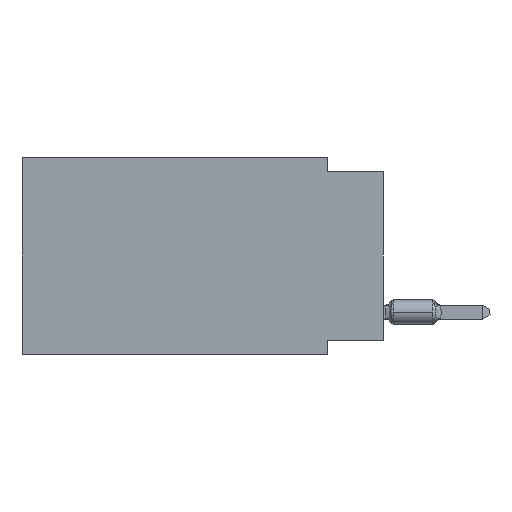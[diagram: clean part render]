
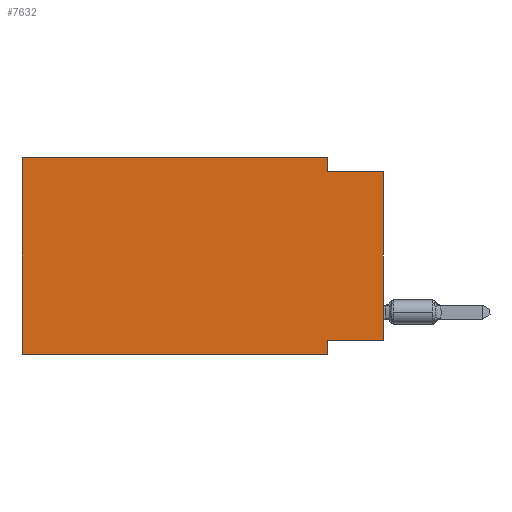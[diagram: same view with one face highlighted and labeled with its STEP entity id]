
A CAD part, left-side view. The second image highlights one B-rep face of the part: STEP entity #7632.
In plain terms, the highlighted planar face has unit normal (-1, 0, 0).
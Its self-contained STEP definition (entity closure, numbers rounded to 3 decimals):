
#23 = EDGE_CURVE ( 'NONE', #9929, #15581, #19994, .T. ) ;
#679 = ORIENTED_EDGE ( 'NONE', *, *, #10187, .F. ) ;
#808 = VECTOR ( 'NONE', #7598, 1000. ) ;
#1377 = ORIENTED_EDGE ( 'NONE', *, *, #15057, .F. ) ;
#1378 = LINE ( 'NONE', #15219, #3775 ) ;
#1688 = CARTESIAN_POINT ( 'NONE',  ( 0., 0., -8.255 ) ) ;
#1739 = VECTOR ( 'NONE', #7626, 1000. ) ;
#1839 = EDGE_CURVE ( 'NONE', #20794, #7504, #7367, .T. ) ;
#2128 = VECTOR ( 'NONE', #15510, 1000. ) ;
#2418 = LINE ( 'NONE', #11044, #1739 ) ;
#3391 = DIRECTION ( 'NONE',  ( 1., 0., 0. ) ) ;
#3775 = VECTOR ( 'NONE', #20628, 1000. ) ;
#4055 = CARTESIAN_POINT ( 'NONE',  ( 0., 2.54, 0. ) ) ;
#4470 = CARTESIAN_POINT ( 'NONE',  ( 0., 2.54, -8.89 ) ) ;
#5055 = DIRECTION ( 'NONE',  ( 0., 0., -1. ) ) ;
#5067 = CARTESIAN_POINT ( 'NONE',  ( 0., 16.383, 0. ) ) ;
#5190 = PLANE ( 'NONE',  #21615 ) ;
#5310 = EDGE_CURVE ( 'NONE', #8662, #15581, #6787, .T. ) ;
#5370 = VERTEX_POINT ( 'NONE', #14698 ) ;
#5507 = VECTOR ( 'NONE', #5919, 1000. ) ;
#5919 = DIRECTION ( 'NONE',  ( 0., 1., 0. ) ) ;
#6044 = EDGE_CURVE ( 'NONE', #9859, #20794, #20793, .T. ) ;
#6668 = CARTESIAN_POINT ( 'NONE',  ( 0., 2.54, -8.89 ) ) ;
#6787 = LINE ( 'NONE', #10658, #808 ) ;
#7367 = LINE ( 'NONE', #9318, #22335 ) ;
#7504 = VERTEX_POINT ( 'NONE', #9598 ) ;
#7598 = DIRECTION ( 'NONE',  ( 0., -1., 0. ) ) ;
#7626 = DIRECTION ( 'NONE',  ( 0., 0., 1. ) ) ;
#7632 = ADVANCED_FACE ( 'NONE', ( #22309 ), #5190, .F. ) ;
#8662 = VERTEX_POINT ( 'NONE', #16395 ) ;
#8968 = VECTOR ( 'NONE', #5055, 1000. ) ;
#9025 = EDGE_CURVE ( 'NONE', #22347, #7504, #2418, .T. ) ;
#9310 = VECTOR ( 'NONE', #19646, 1000. ) ;
#9318 = CARTESIAN_POINT ( 'NONE',  ( 0., 0., -0.635 ) ) ;
#9598 = CARTESIAN_POINT ( 'NONE',  ( 0., 0., -0.635 ) ) ;
#9849 = ORIENTED_EDGE ( 'NONE', *, *, #1839, .F. ) ;
#9859 = VERTEX_POINT ( 'NONE', #4055 ) ;
#9929 = VERTEX_POINT ( 'NONE', #18569 ) ;
#10187 = EDGE_CURVE ( 'NONE', #8662, #5370, #12223, .T. ) ;
#10658 = CARTESIAN_POINT ( 'NONE',  ( 0., 16.383, -8.89 ) ) ;
#11044 = CARTESIAN_POINT ( 'NONE',  ( 0., 0., 0. ) ) ;
#12223 = LINE ( 'NONE', #5067, #2128 ) ;
#12614 = DIRECTION ( 'NONE',  ( 0., -1., 0. ) ) ;
#13385 = CARTESIAN_POINT ( 'NONE',  ( 0., 2.54, -0.635 ) ) ;
#13577 = CARTESIAN_POINT ( 'NONE',  ( 0., 2.54, 0. ) ) ;
#13889 = ORIENTED_EDGE ( 'NONE', *, *, #23, .F. ) ;
#14146 = CARTESIAN_POINT ( 'NONE',  ( 0., 16.383, 0. ) ) ;
#14698 = CARTESIAN_POINT ( 'NONE',  ( 0., 16.383, 0. ) ) ;
#15057 = EDGE_CURVE ( 'NONE', #22347, #9929, #21437, .T. ) ;
#15219 = CARTESIAN_POINT ( 'NONE',  ( 0., 16.383, 0. ) ) ;
#15510 = DIRECTION ( 'NONE',  ( 0., 0., 1. ) ) ;
#15581 = VERTEX_POINT ( 'NONE', #6668 ) ;
#16395 = CARTESIAN_POINT ( 'NONE',  ( 0., 16.383, -8.89 ) ) ;
#16597 = CARTESIAN_POINT ( 'NONE',  ( 0., 0., -8.255 ) ) ;
#17402 = ORIENTED_EDGE ( 'NONE', *, *, #5310, .T. ) ;
#17545 = ORIENTED_EDGE ( 'NONE', *, *, #6044, .F. ) ;
#18569 = CARTESIAN_POINT ( 'NONE',  ( 0., 2.54, -8.255 ) ) ;
#19237 = ORIENTED_EDGE ( 'NONE', *, *, #9025, .T. ) ;
#19646 = DIRECTION ( 'NONE',  ( 0., 0., -1. ) ) ;
#19994 = LINE ( 'NONE', #4470, #9310 ) ;
#20453 = EDGE_CURVE ( 'NONE', #5370, #9859, #1378, .T. ) ;
#20628 = DIRECTION ( 'NONE',  ( 0., -1., 0. ) ) ;
#20710 = DIRECTION ( 'NONE',  ( 0., 0., -1. ) ) ;
#20793 = LINE ( 'NONE', #13577, #8968 ) ;
#20794 = VERTEX_POINT ( 'NONE', #13385 ) ;
#20909 = EDGE_LOOP ( 'NONE', ( #19237, #9849, #17545, #21379, #679, #17402, #13889, #1377 ) ) ;
#21379 = ORIENTED_EDGE ( 'NONE', *, *, #20453, .F. ) ;
#21437 = LINE ( 'NONE', #16597, #5507 ) ;
#21615 = AXIS2_PLACEMENT_3D ( 'NONE', #14146, #3391, #20710 ) ;
#22309 = FACE_OUTER_BOUND ( 'NONE', #20909, .T. ) ;
#22335 = VECTOR ( 'NONE', #12614, 1000. ) ;
#22347 = VERTEX_POINT ( 'NONE', #1688 ) ;
